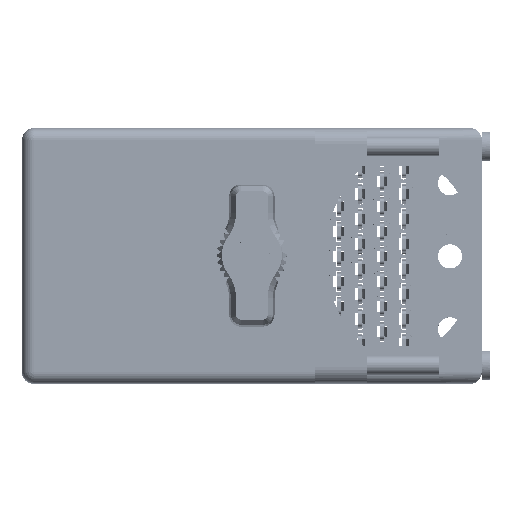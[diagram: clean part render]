
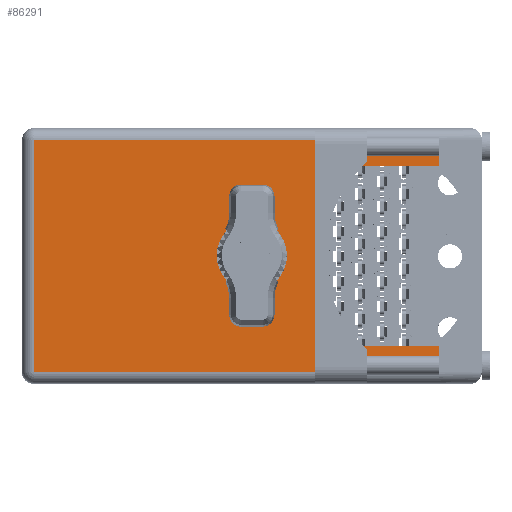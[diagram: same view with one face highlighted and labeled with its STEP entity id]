
A CAD part, top view. The second image highlights one B-rep face of the part: STEP entity #86291.
In plain terms, the highlighted face is planar.
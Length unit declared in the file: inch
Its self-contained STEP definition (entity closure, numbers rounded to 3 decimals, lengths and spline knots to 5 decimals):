
#1311 = VERTEX_POINT ( 'NONE', #92295 ) ;
#4844 = ORIENTED_EDGE ( 'NONE', *, *, #59795, .T. ) ;
#6727 = LINE ( 'NONE', #47701, #41947 ) ;
#6958 = CARTESIAN_POINT ( 'NONE',  ( 2.499, 2.03, -1.305 ) ) ;
#7804 = DIRECTION ( 'NONE',  ( -1., 0., 0. ) ) ;
#8495 = LINE ( 'NONE', #25637, #95192 ) ;
#9551 = CARTESIAN_POINT ( 'NONE',  ( 1.785, 2.03, -1.305 ) ) ;
#9880 = EDGE_CURVE ( 'NONE', #104056, #104383, #41886, .T. ) ;
#11717 = ORIENTED_EDGE ( 'NONE', *, *, #19489, .F. ) ;
#13802 = VERTEX_POINT ( 'NONE', #83134 ) ;
#14314 = LINE ( 'NONE', #73562, #34735 ) ;
#15344 = CARTESIAN_POINT ( 'NONE',  ( 2.499, 2.03, -1.305 ) ) ;
#15353 = DIRECTION ( 'NONE',  ( 0., 1., 0. ) ) ;
#15733 = LINE ( 'NONE', #108184, #93051 ) ;
#16225 = EDGE_LOOP ( 'NONE', ( #11717, #97740 ) ) ;
#17838 = DIRECTION ( 'NONE',  ( 0., 1., 0. ) ) ;
#18389 = FACE_OUTER_BOUND ( 'NONE', #31654, .T. ) ;
#19489 = EDGE_CURVE ( 'NONE', #54587, #37692, #95784, .T. ) ;
#20938 = ORIENTED_EDGE ( 'NONE', *, *, #70671, .T. ) ;
#22813 = ORIENTED_EDGE ( 'NONE', *, *, #25015, .F. ) ;
#25015 = EDGE_CURVE ( 'NONE', #51203, #13802, #74965, .T. ) ;
#25030 = CIRCLE ( 'NONE', #101030, 0.17 ) ;
#25313 = CARTESIAN_POINT ( 'NONE',  ( 2.499, 2.03, -1.46 ) ) ;
#25637 = CARTESIAN_POINT ( 'NONE',  ( 0., 2.03, -1.46 ) ) ;
#27196 = CARTESIAN_POINT ( 'NONE',  ( 2.499, 2.03, -0.225 ) ) ;
#27560 = VECTOR ( 'NONE', #51815, 39.37008 ) ;
#29546 = DIRECTION ( 'NONE',  ( 0., 1., 0. ) ) ;
#31654 = EDGE_LOOP ( 'NONE', ( #75641, #90847, #22813, #20938, #66420, #79196, #65142, #4844 ) ) ;
#33102 = DIRECTION ( 'NONE',  ( 0., 0., 1. ) ) ;
#34443 = CARTESIAN_POINT ( 'NONE',  ( 0., 2.03, -1.53 ) ) ;
#34637 = CARTESIAN_POINT ( 'NONE',  ( 2.499, 2.03, -1.53 ) ) ;
#34735 = VECTOR ( 'NONE', #33102, 39.37008 ) ;
#34996 = DIRECTION ( 'NONE',  ( 0., 0., -1. ) ) ;
#37692 = VERTEX_POINT ( 'NONE', #106662 ) ;
#39710 = EDGE_CURVE ( 'NONE', #76664, #13802, #15733, .T. ) ;
#40083 = DIRECTION ( 'NONE',  ( -1., 0., 0. ) ) ;
#41886 = LINE ( 'NONE', #34637, #27560 ) ;
#41947 = VECTOR ( 'NONE', #7804, 39.37008 ) ;
#47701 = CARTESIAN_POINT ( 'NONE',  ( 2.499, 2.03, -0.225 ) ) ;
#48106 = AXIS2_PLACEMENT_3D ( 'NONE', #58002, #15353, #90097 ) ;
#49394 = VECTOR ( 'NONE', #101102, 39.37008 ) ;
#49535 = DIRECTION ( 'NONE',  ( 1., 0., 0. ) ) ;
#50077 = EDGE_CURVE ( 'NONE', #1311, #104383, #82357, .T. ) ;
#50569 = VERTEX_POINT ( 'NONE', #108197 ) ;
#51203 = VERTEX_POINT ( 'NONE', #27196 ) ;
#51815 = DIRECTION ( 'NONE',  ( 0., 0., 1. ) ) ;
#52160 = PLANE ( 'NONE',  #61523 ) ;
#54587 = VERTEX_POINT ( 'NONE', #54634 ) ;
#54634 = CARTESIAN_POINT ( 'NONE',  ( 1.3775, 2.03, -0.595 ) ) ;
#55215 = VECTOR ( 'NONE', #108711, 39.37008 ) ;
#58002 = CARTESIAN_POINT ( 'NONE',  ( 1.3775, 2.03, -0.765 ) ) ;
#58841 = LINE ( 'NONE', #9551, #60446 ) ;
#59795 = EDGE_CURVE ( 'NONE', #104056, #50569, #8495, .T. ) ;
#60446 = VECTOR ( 'NONE', #34996, 39.37008 ) ;
#61523 = AXIS2_PLACEMENT_3D ( 'NONE', #34443, #17838, #85913 ) ;
#63545 = EDGE_CURVE ( 'NONE', #37692, #54587, #25030, .T. ) ;
#65142 = ORIENTED_EDGE ( 'NONE', *, *, #9880, .F. ) ;
#66420 = ORIENTED_EDGE ( 'NONE', *, *, #106263, .T. ) ;
#70556 = DIRECTION ( 'NONE',  ( 0., 0., 1. ) ) ;
#70671 = EDGE_CURVE ( 'NONE', #51203, #108751, #6727, .T. ) ;
#73562 = CARTESIAN_POINT ( 'NONE',  ( 0.07, 2.03, -1.53 ) ) ;
#74428 = CARTESIAN_POINT ( 'NONE',  ( 2.499, 2.03, -1.53 ) ) ;
#74965 = LINE ( 'NONE', #74428, #55215 ) ;
#75641 = ORIENTED_EDGE ( 'NONE', *, *, #80001, .T. ) ;
#76664 = VERTEX_POINT ( 'NONE', #107018 ) ;
#79196 = ORIENTED_EDGE ( 'NONE', *, *, #50077, .T. ) ;
#79410 = CARTESIAN_POINT ( 'NONE',  ( 1.3775, 2.03, -0.765 ) ) ;
#80001 = EDGE_CURVE ( 'NONE', #50569, #76664, #14314, .T. ) ;
#82357 = LINE ( 'NONE', #15344, #49394 ) ;
#83134 = CARTESIAN_POINT ( 'NONE',  ( 2.499, 2.03, -0.07 ) ) ;
#85913 = DIRECTION ( 'NONE',  ( 0., 0., 1. ) ) ;
#86291 = ADVANCED_FACE ( 'NONE', ( #18389, #95294 ), #52160, .T. ) ;
#90097 = DIRECTION ( 'NONE',  ( 0., 0., 1. ) ) ;
#90847 = ORIENTED_EDGE ( 'NONE', *, *, #39710, .T. ) ;
#92295 = CARTESIAN_POINT ( 'NONE',  ( 1.785, 2.03, -1.305 ) ) ;
#93051 = VECTOR ( 'NONE', #49535, 39.37008 ) ;
#95192 = VECTOR ( 'NONE', #40083, 39.37008 ) ;
#95294 = FACE_BOUND ( 'NONE', #16225, .T. ) ;
#95784 = CIRCLE ( 'NONE', #48106, 0.17 ) ;
#97740 = ORIENTED_EDGE ( 'NONE', *, *, #63545, .F. ) ;
#101030 = AXIS2_PLACEMENT_3D ( 'NONE', #79410, #29546, #70556 ) ;
#101102 = DIRECTION ( 'NONE',  ( 1., 0., 0. ) ) ;
#103235 = CARTESIAN_POINT ( 'NONE',  ( 1.785, 2.03, -0.225 ) ) ;
#104056 = VERTEX_POINT ( 'NONE', #25313 ) ;
#104383 = VERTEX_POINT ( 'NONE', #6958 ) ;
#106263 = EDGE_CURVE ( 'NONE', #108751, #1311, #58841, .T. ) ;
#106662 = CARTESIAN_POINT ( 'NONE',  ( 1.3775, 2.03, -0.935 ) ) ;
#107018 = CARTESIAN_POINT ( 'NONE',  ( 0.07, 2.03, -0.07 ) ) ;
#108184 = CARTESIAN_POINT ( 'NONE',  ( 2.499, 2.03, -0.07 ) ) ;
#108197 = CARTESIAN_POINT ( 'NONE',  ( 0.07, 2.03, -1.46 ) ) ;
#108711 = DIRECTION ( 'NONE',  ( 0., 0., 1. ) ) ;
#108751 = VERTEX_POINT ( 'NONE', #103235 ) ;
